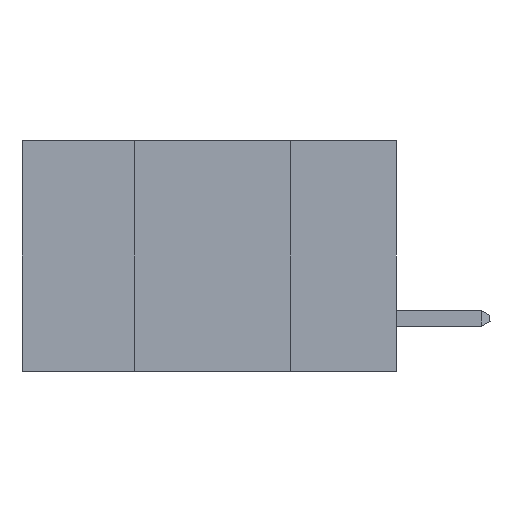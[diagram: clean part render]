
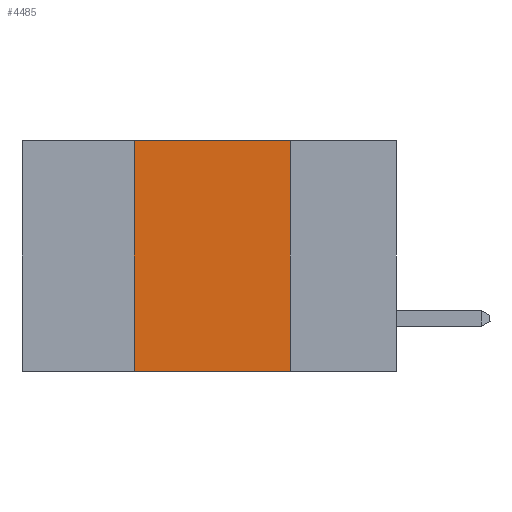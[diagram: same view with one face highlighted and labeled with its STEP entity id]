
A CAD part, left-side view. The second image highlights one B-rep face of the part: STEP entity #4485.
In plain terms, the highlighted planar face has unit normal (-1, 0, 0).
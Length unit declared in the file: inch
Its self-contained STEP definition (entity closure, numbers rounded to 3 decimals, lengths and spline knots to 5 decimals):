
#218 = CARTESIAN_POINT ( 'NONE',  ( 0., 0.42, 0. ) ) ;
#1436 = DIRECTION ( 'NONE',  ( 0., 0., 1. ) ) ;
#1693 = DIRECTION ( 'NONE',  ( 0., 0., -1. ) ) ;
#2011 = CARTESIAN_POINT ( 'NONE',  ( 0., 0.42, -0.37 ) ) ;
#2035 = LINE ( 'NONE', #218, #11220 ) ;
#2538 = VERTEX_POINT ( 'NONE', #5192 ) ;
#2575 = AXIS2_PLACEMENT_3D ( 'NONE', #9667, #9130, #7095 ) ;
#3719 = EDGE_LOOP ( 'NONE', ( #7825, #14903, #15089, #7647 ) ) ;
#3748 = LINE ( 'NONE', #10858, #9802 ) ;
#4295 = CARTESIAN_POINT ( 'NONE',  ( 0., 0.42, 0. ) ) ;
#4485 = ADVANCED_FACE ( 'NONE', ( #6442 ), #10984, .F. ) ;
#4632 = VERTEX_POINT ( 'NONE', #9966 ) ;
#5043 = EDGE_CURVE ( 'NONE', #13583, #2538, #7364, .T. ) ;
#5192 = CARTESIAN_POINT ( 'NONE',  ( 0., 0.17, 0. ) ) ;
#5905 = VECTOR ( 'NONE', #1693, 39.37008 ) ;
#6442 = FACE_OUTER_BOUND ( 'NONE', #3719, .T. ) ;
#7095 = DIRECTION ( 'NONE',  ( 0., 0., -1. ) ) ;
#7364 = LINE ( 'NONE', #13890, #12897 ) ;
#7647 = ORIENTED_EDGE ( 'NONE', *, *, #12613, .T. ) ;
#7744 = CARTESIAN_POINT ( 'NONE',  ( 0., 0.17, 0. ) ) ;
#7825 = ORIENTED_EDGE ( 'NONE', *, *, #14121, .F. ) ;
#9130 = DIRECTION ( 'NONE',  ( 1., 0., 0. ) ) ;
#9142 = VERTEX_POINT ( 'NONE', #2011 ) ;
#9667 = CARTESIAN_POINT ( 'NONE',  ( 0., 0.6, 0. ) ) ;
#9802 = VECTOR ( 'NONE', #12067, 39.37008 ) ;
#9966 = CARTESIAN_POINT ( 'NONE',  ( 0., 0.17, -0.37 ) ) ;
#10858 = CARTESIAN_POINT ( 'NONE',  ( 0., 0.6, -0.37 ) ) ;
#10984 = PLANE ( 'NONE',  #2575 ) ;
#11220 = VECTOR ( 'NONE', #1436, 39.37008 ) ;
#12067 = DIRECTION ( 'NONE',  ( 0., -1., 0. ) ) ;
#12608 = LINE ( 'NONE', #7744, #5905 ) ;
#12613 = EDGE_CURVE ( 'NONE', #9142, #4632, #3748, .T. ) ;
#12897 = VECTOR ( 'NONE', #13902, 39.37008 ) ;
#13356 = EDGE_CURVE ( 'NONE', #9142, #13583, #2035, .T. ) ;
#13583 = VERTEX_POINT ( 'NONE', #4295 ) ;
#13890 = CARTESIAN_POINT ( 'NONE',  ( 0., 0.6, 0. ) ) ;
#13902 = DIRECTION ( 'NONE',  ( 0., -1., 0. ) ) ;
#14121 = EDGE_CURVE ( 'NONE', #2538, #4632, #12608, .T. ) ;
#14903 = ORIENTED_EDGE ( 'NONE', *, *, #5043, .F. ) ;
#15089 = ORIENTED_EDGE ( 'NONE', *, *, #13356, .F. ) ;
